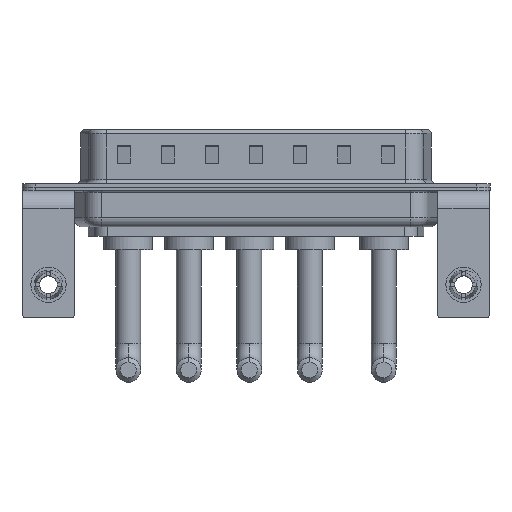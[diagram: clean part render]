
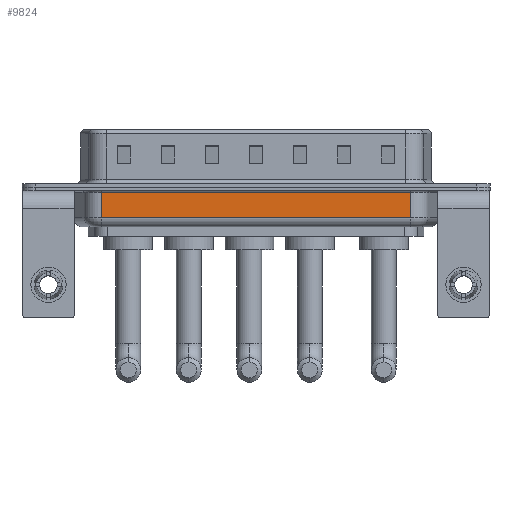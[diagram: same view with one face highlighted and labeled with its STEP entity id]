
A CAD part, front view. The second image highlights one B-rep face of the part: STEP entity #9824.
In plain terms, the highlighted planar face has unit normal (0, -1, 0).
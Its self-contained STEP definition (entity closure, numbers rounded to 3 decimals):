
#9 = CARTESIAN_POINT ( 'NONE',  ( 6.006, -5.35, -4.5 ) ) ;
#590 = EDGE_CURVE ( 'NONE', #10899, #15858, #1920, .T. ) ;
#626 = EDGE_CURVE ( 'NONE', #15357, #10899, #16181, .T. ) ;
#832 = AXIS2_PLACEMENT_3D ( 'NONE', #6426, #8725, #6178 ) ;
#914 = FACE_OUTER_BOUND ( 'NONE', #3766, .T. ) ;
#1126 = DIRECTION ( 'NONE',  ( 1., 0., 0. ) ) ;
#1721 = CARTESIAN_POINT ( 'NONE',  ( 41.044, -5.35, -3.5 ) ) ;
#1920 = LINE ( 'NONE', #9651, #16449 ) ;
#2347 = PLANE ( 'NONE',  #832 ) ;
#2512 = VECTOR ( 'NONE', #1126, 1000. ) ;
#2712 = LINE ( 'NONE', #9, #10516 ) ;
#3531 = VERTEX_POINT ( 'NONE', #10944 ) ;
#3580 = CARTESIAN_POINT ( 'NONE',  ( 6.006, -5.35, -3.5 ) ) ;
#3766 = EDGE_LOOP ( 'NONE', ( #14044, #11564, #4470, #3826 ) ) ;
#3826 = ORIENTED_EDGE ( 'NONE', *, *, #590, .T. ) ;
#4470 = ORIENTED_EDGE ( 'NONE', *, *, #626, .T. ) ;
#4865 = LINE ( 'NONE', #3580, #2512 ) ;
#5179 = DIRECTION ( 'NONE',  ( 0., 0., 1. ) ) ;
#5508 = CARTESIAN_POINT ( 'NONE',  ( 41.044, -5.35, -0.65 ) ) ;
#5738 = DIRECTION ( 'NONE',  ( 0., 0., 1. ) ) ;
#6080 = CARTESIAN_POINT ( 'NONE',  ( 41.044, -5.35, -4.5 ) ) ;
#6178 = DIRECTION ( 'NONE',  ( 0., 0., 1. ) ) ;
#6426 = CARTESIAN_POINT ( 'NONE',  ( 6.006, -5.35, -4.5 ) ) ;
#7416 = EDGE_CURVE ( 'NONE', #3531, #15858, #2712, .T. ) ;
#8725 = DIRECTION ( 'NONE',  ( 0., 1., 0. ) ) ;
#9651 = CARTESIAN_POINT ( 'NONE',  ( 6.006, -5.35, -0.65 ) ) ;
#9824 = ADVANCED_FACE ( 'NONE', ( #914 ), #2347, .F. ) ;
#10516 = VECTOR ( 'NONE', #5179, 1000. ) ;
#10899 = VERTEX_POINT ( 'NONE', #5508 ) ;
#10944 = CARTESIAN_POINT ( 'NONE',  ( 6.006, -5.35, -3.5 ) ) ;
#11564 = ORIENTED_EDGE ( 'NONE', *, *, #12207, .T. ) ;
#12207 = EDGE_CURVE ( 'NONE', #3531, #15357, #4865, .T. ) ;
#12982 = CARTESIAN_POINT ( 'NONE',  ( 6.006, -5.35, -0.65 ) ) ;
#13553 = DIRECTION ( 'NONE',  ( -1., 0., 0. ) ) ;
#14044 = ORIENTED_EDGE ( 'NONE', *, *, #7416, .F. ) ;
#15357 = VERTEX_POINT ( 'NONE', #1721 ) ;
#15858 = VERTEX_POINT ( 'NONE', #12982 ) ;
#15964 = VECTOR ( 'NONE', #5738, 1000. ) ;
#16181 = LINE ( 'NONE', #6080, #15964 ) ;
#16449 = VECTOR ( 'NONE', #13553, 1000. ) ;
